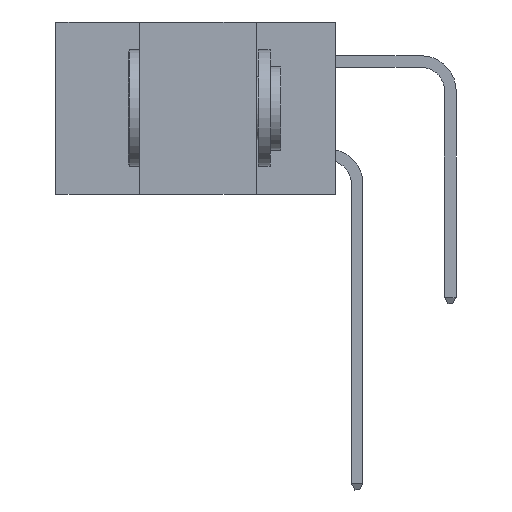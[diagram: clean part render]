
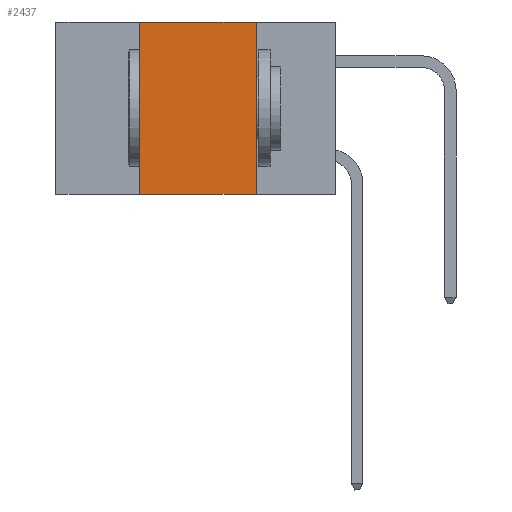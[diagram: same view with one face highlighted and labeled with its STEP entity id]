
A CAD part, left-side view. The second image highlights one B-rep face of the part: STEP entity #2437.
In plain terms, the highlighted planar face has unit normal (-1, 0, 0).
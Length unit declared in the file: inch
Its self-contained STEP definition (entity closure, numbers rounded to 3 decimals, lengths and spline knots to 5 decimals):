
#1783 = VECTOR ( 'NONE', #2260, 39.37008 ) ;
#1911 = CARTESIAN_POINT ( 'NONE',  ( 0., 0.6, -0.37 ) ) ;
#1993 = FACE_OUTER_BOUND ( 'NONE', #2408, .T. ) ;
#1999 = CARTESIAN_POINT ( 'NONE',  ( 0., 0.17, -0.37 ) ) ;
#2260 = DIRECTION ( 'NONE',  ( 0., -1., 0. ) ) ;
#2408 = EDGE_LOOP ( 'NONE', ( #9936, #9966, #10357, #10802 ) ) ;
#2435 = EDGE_CURVE ( 'NONE', #7565, #7977, #11049, .T. ) ;
#2437 = ADVANCED_FACE ( 'NONE', ( #1993 ), #3051, .F. ) ;
#3051 = PLANE ( 'NONE',  #7410 ) ;
#3134 = DIRECTION ( 'NONE',  ( 0., -1., 0. ) ) ;
#4707 = CARTESIAN_POINT ( 'NONE',  ( 0., 0.42, -0.37 ) ) ;
#5016 = VECTOR ( 'NONE', #3134, 39.37008 ) ;
#5150 = VECTOR ( 'NONE', #6970, 39.37008 ) ;
#5971 = LINE ( 'NONE', #10136, #8662 ) ;
#6768 = CARTESIAN_POINT ( 'NONE',  ( 0., 0.6, 0. ) ) ;
#6925 = CARTESIAN_POINT ( 'NONE',  ( 0., 0.42, 0. ) ) ;
#6970 = DIRECTION ( 'NONE',  ( 0., 0., -1. ) ) ;
#7410 = AXIS2_PLACEMENT_3D ( 'NONE', #10810, #12497, #14444 ) ;
#7434 = EDGE_CURVE ( 'NONE', #7565, #13614, #5971, .T. ) ;
#7456 = LINE ( 'NONE', #6768, #1783 ) ;
#7565 = VERTEX_POINT ( 'NONE', #4707 ) ;
#7977 = VERTEX_POINT ( 'NONE', #1999 ) ;
#8662 = VECTOR ( 'NONE', #12357, 39.37008 ) ;
#9936 = ORIENTED_EDGE ( 'NONE', *, *, #12683, .F. ) ;
#9966 = ORIENTED_EDGE ( 'NONE', *, *, #13535, .F. ) ;
#10136 = CARTESIAN_POINT ( 'NONE',  ( 0., 0.42, 0. ) ) ;
#10357 = ORIENTED_EDGE ( 'NONE', *, *, #7434, .F. ) ;
#10802 = ORIENTED_EDGE ( 'NONE', *, *, #2435, .T. ) ;
#10810 = CARTESIAN_POINT ( 'NONE',  ( 0., 0.6, 0. ) ) ;
#11049 = LINE ( 'NONE', #1911, #5016 ) ;
#11180 = LINE ( 'NONE', #13644, #5150 ) ;
#11547 = VERTEX_POINT ( 'NONE', #12553 ) ;
#12357 = DIRECTION ( 'NONE',  ( 0., 0., 1. ) ) ;
#12497 = DIRECTION ( 'NONE',  ( 1., 0., 0. ) ) ;
#12553 = CARTESIAN_POINT ( 'NONE',  ( 0., 0.17, 0. ) ) ;
#12683 = EDGE_CURVE ( 'NONE', #11547, #7977, #11180, .T. ) ;
#13535 = EDGE_CURVE ( 'NONE', #13614, #11547, #7456, .T. ) ;
#13614 = VERTEX_POINT ( 'NONE', #6925 ) ;
#13644 = CARTESIAN_POINT ( 'NONE',  ( 0., 0.17, 0. ) ) ;
#14444 = DIRECTION ( 'NONE',  ( 0., 0., -1. ) ) ;
